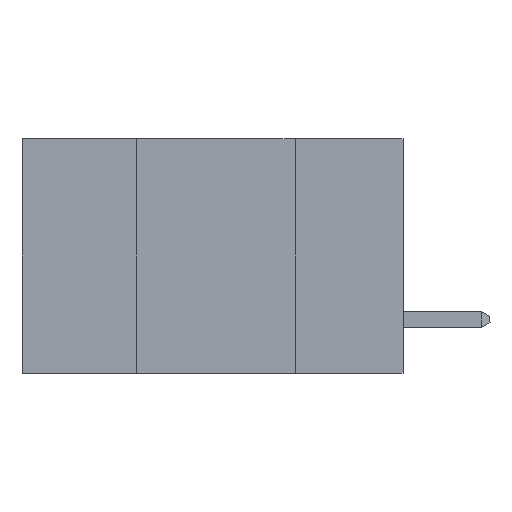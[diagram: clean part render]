
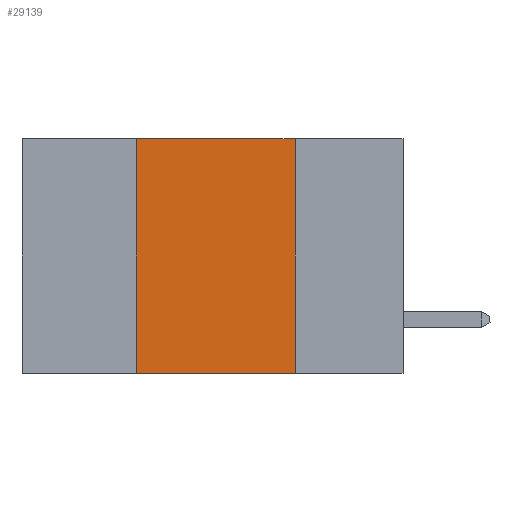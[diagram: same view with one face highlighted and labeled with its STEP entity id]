
A CAD part, left-side view. The second image highlights one B-rep face of the part: STEP entity #29139.
In plain terms, the highlighted planar face has unit normal (-1, 0, 0).
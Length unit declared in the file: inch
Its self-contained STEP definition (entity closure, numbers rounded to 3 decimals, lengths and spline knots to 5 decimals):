
#1677 = VERTEX_POINT ( 'NONE', #23536 ) ;
#2293 = PLANE ( 'NONE',  #15189 ) ;
#2791 = ORIENTED_EDGE ( 'NONE', *, *, #6055, .T. ) ;
#3535 = EDGE_CURVE ( 'NONE', #1677, #18690, #10310, .T. ) ;
#3826 = VECTOR ( 'NONE', #6334, 39.37008 ) ;
#5413 = EDGE_CURVE ( 'NONE', #26088, #1677, #26674, .T. ) ;
#6055 = EDGE_CURVE ( 'NONE', #26088, #12760, #14729, .T. ) ;
#6334 = DIRECTION ( 'NONE',  ( 0., -1., 0. ) ) ;
#6780 = VECTOR ( 'NONE', #30160, 39.37008 ) ;
#9342 = DIRECTION ( 'NONE',  ( 0., 0., 1. ) ) ;
#9404 = CARTESIAN_POINT ( 'NONE',  ( 0., 0.17, 0. ) ) ;
#10310 = LINE ( 'NONE', #16170, #3826 ) ;
#12116 = DIRECTION ( 'NONE',  ( 0., 0., -1. ) ) ;
#12760 = VERTEX_POINT ( 'NONE', #22425 ) ;
#12979 = CARTESIAN_POINT ( 'NONE',  ( 0., 0.17, 0. ) ) ;
#13067 = FACE_OUTER_BOUND ( 'NONE', #16152, .T. ) ;
#14308 = ORIENTED_EDGE ( 'NONE', *, *, #5413, .F. ) ;
#14400 = VECTOR ( 'NONE', #9342, 39.37008 ) ;
#14729 = LINE ( 'NONE', #24596, #26251 ) ;
#15189 = AXIS2_PLACEMENT_3D ( 'NONE', #21923, #26836, #12116 ) ;
#16152 = EDGE_LOOP ( 'NONE', ( #25319, #16930, #14308, #2791 ) ) ;
#16170 = CARTESIAN_POINT ( 'NONE',  ( 0., 0.6, 0. ) ) ;
#16881 = CARTESIAN_POINT ( 'NONE',  ( 0., 0.42, -0.37 ) ) ;
#16930 = ORIENTED_EDGE ( 'NONE', *, *, #3535, .F. ) ;
#18690 = VERTEX_POINT ( 'NONE', #9404 ) ;
#20675 = LINE ( 'NONE', #12979, #6780 ) ;
#21923 = CARTESIAN_POINT ( 'NONE',  ( 0., 0.6, 0. ) ) ;
#22425 = CARTESIAN_POINT ( 'NONE',  ( 0., 0.17, -0.37 ) ) ;
#23536 = CARTESIAN_POINT ( 'NONE',  ( 0., 0.42, 0. ) ) ;
#24596 = CARTESIAN_POINT ( 'NONE',  ( 0., 0.6, -0.37 ) ) ;
#25319 = ORIENTED_EDGE ( 'NONE', *, *, #31665, .F. ) ;
#26088 = VERTEX_POINT ( 'NONE', #16881 ) ;
#26251 = VECTOR ( 'NONE', #27033, 39.37008 ) ;
#26674 = LINE ( 'NONE', #31430, #14400 ) ;
#26836 = DIRECTION ( 'NONE',  ( 1., 0., 0. ) ) ;
#27033 = DIRECTION ( 'NONE',  ( 0., -1., 0. ) ) ;
#29139 = ADVANCED_FACE ( 'NONE', ( #13067 ), #2293, .F. ) ;
#30160 = DIRECTION ( 'NONE',  ( 0., 0., -1. ) ) ;
#31430 = CARTESIAN_POINT ( 'NONE',  ( 0., 0.42, 0. ) ) ;
#31665 = EDGE_CURVE ( 'NONE', #18690, #12760, #20675, .T. ) ;
